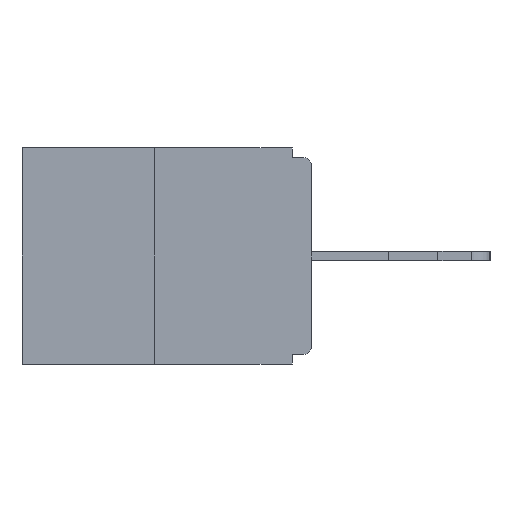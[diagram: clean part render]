
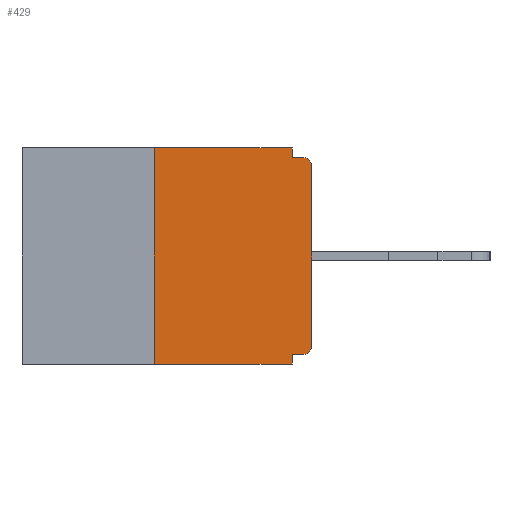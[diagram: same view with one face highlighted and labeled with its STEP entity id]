
A CAD part, left-side view. The second image highlights one B-rep face of the part: STEP entity #429.
In plain terms, the highlighted planar face has unit normal (-1, 0, 0).
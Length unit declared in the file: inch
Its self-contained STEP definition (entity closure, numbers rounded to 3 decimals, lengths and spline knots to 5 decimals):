
#134 = VERTEX_POINT ( 'NONE', #3484 ) ;
#415 = CARTESIAN_POINT ( 'NONE',  ( 0., 0.46, 0. ) ) ;
#429 = ADVANCED_FACE ( 'NONE', ( #4463 ), #9587, .F. ) ;
#510 = EDGE_CURVE ( 'NONE', #134, #20403, #24511, .T. ) ;
#675 = VECTOR ( 'NONE', #11992, 39.37008 ) ;
#1429 = DIRECTION ( 'NONE',  ( 1., 0., 0. ) ) ;
#1517 = DIRECTION ( 'NONE',  ( 0., 1., 0. ) ) ;
#1575 = EDGE_CURVE ( 'NONE', #20032, #6018, #9536, .T. ) ;
#1685 = CARTESIAN_POINT ( 'NONE',  ( 0., 0.46, -0.343 ) ) ;
#1712 = CARTESIAN_POINT ( 'NONE',  ( 0., 0.015, -0.313 ) ) ;
#1956 = CARTESIAN_POINT ( 'NONE',  ( 0., 0., -0.015 ) ) ;
#2131 = LINE ( 'NONE', #18532, #675 ) ;
#2180 = CARTESIAN_POINT ( 'NONE',  ( 0., 0., -0.313 ) ) ;
#2469 = EDGE_CURVE ( 'NONE', #26115, #7521, #4935, .T. ) ;
#3102 = DIRECTION ( 'NONE',  ( 0., -1., 0. ) ) ;
#3484 = CARTESIAN_POINT ( 'NONE',  ( 0., 0., -0.03 ) ) ;
#3559 = VECTOR ( 'NONE', #7073, 39.37008 ) ;
#4042 = DIRECTION ( 'NONE',  ( 0., 0., -1. ) ) ;
#4463 = FACE_OUTER_BOUND ( 'NONE', #23758, .T. ) ;
#4718 = LINE ( 'NONE', #1956, #21515 ) ;
#4935 = LINE ( 'NONE', #19039, #9870 ) ;
#4983 = ORIENTED_EDGE ( 'NONE', *, *, #21768, .T. ) ;
#4991 = VERTEX_POINT ( 'NONE', #2180 ) ;
#5872 = CARTESIAN_POINT ( 'NONE',  ( 0., 0.031, 0. ) ) ;
#6018 = VERTEX_POINT ( 'NONE', #18554 ) ;
#6286 = ORIENTED_EDGE ( 'NONE', *, *, #24197, .T. ) ;
#6769 = EDGE_CURVE ( 'NONE', #26792, #20403, #4718, .T. ) ;
#6835 = ORIENTED_EDGE ( 'NONE', *, *, #510, .T. ) ;
#6921 = EDGE_CURVE ( 'NONE', #4991, #134, #27020, .T. ) ;
#7037 = ORIENTED_EDGE ( 'NONE', *, *, #6769, .F. ) ;
#7073 = DIRECTION ( 'NONE',  ( 0., 0., -1. ) ) ;
#7521 = VERTEX_POINT ( 'NONE', #11473 ) ;
#8380 = CARTESIAN_POINT ( 'NONE',  ( 0., 0., -0.328 ) ) ;
#9536 = LINE ( 'NONE', #11171, #3559 ) ;
#9587 = PLANE ( 'NONE',  #10452 ) ;
#9870 = VECTOR ( 'NONE', #21928, 39.37008 ) ;
#10041 = ORIENTED_EDGE ( 'NONE', *, *, #2469, .F. ) ;
#10452 = AXIS2_PLACEMENT_3D ( 'NONE', #415, #1429, #25728 ) ;
#10807 = ORIENTED_EDGE ( 'NONE', *, *, #24813, .F. ) ;
#11171 = CARTESIAN_POINT ( 'NONE',  ( 0., 0.031, -0.343 ) ) ;
#11473 = CARTESIAN_POINT ( 'NONE',  ( 0., 0.25, 0. ) ) ;
#11699 = CARTESIAN_POINT ( 'NONE',  ( 0., 0.031, -0.328 ) ) ;
#11858 = ORIENTED_EDGE ( 'NONE', *, *, #15139, .F. ) ;
#11992 = DIRECTION ( 'NONE',  ( 0., -1., 0. ) ) ;
#13559 = ORIENTED_EDGE ( 'NONE', *, *, #6921, .T. ) ;
#13993 = VERTEX_POINT ( 'NONE', #5872 ) ;
#14377 = AXIS2_PLACEMENT_3D ( 'NONE', #1712, #17237, #4042 ) ;
#14824 = AXIS2_PLACEMENT_3D ( 'NONE', #27119, #28222, #25257 ) ;
#15139 = EDGE_CURVE ( 'NONE', #7521, #13993, #2131, .T. ) ;
#15173 = CARTESIAN_POINT ( 'NONE',  ( 0., 0.25, -0.343 ) ) ;
#15733 = VECTOR ( 'NONE', #1517, 39.37008 ) ;
#16503 = LINE ( 'NONE', #23653, #27327 ) ;
#17237 = DIRECTION ( 'NONE',  ( -1., 0., 0. ) ) ;
#18532 = CARTESIAN_POINT ( 'NONE',  ( 0., 0.46, 0. ) ) ;
#18554 = CARTESIAN_POINT ( 'NONE',  ( 0., 0.031, -0.343 ) ) ;
#19039 = CARTESIAN_POINT ( 'NONE',  ( 0., 0.25, 0. ) ) ;
#19692 = CARTESIAN_POINT ( 'NONE',  ( 0., 0.031, -0.015 ) ) ;
#20016 = ORIENTED_EDGE ( 'NONE', *, *, #20927, .F. ) ;
#20032 = VERTEX_POINT ( 'NONE', #11699 ) ;
#20403 = VERTEX_POINT ( 'NONE', #21704 ) ;
#20927 = EDGE_CURVE ( 'NONE', #26843, #20032, #27241, .T. ) ;
#21291 = VECTOR ( 'NONE', #22231, 39.37008 ) ;
#21306 = VECTOR ( 'NONE', #23831, 39.37008 ) ;
#21515 = VECTOR ( 'NONE', #3102, 39.37008 ) ;
#21704 = CARTESIAN_POINT ( 'NONE',  ( 0., 0.015, -0.015 ) ) ;
#21768 = EDGE_CURVE ( 'NONE', #26843, #4991, #25808, .T. ) ;
#21928 = DIRECTION ( 'NONE',  ( 0., 0., 1. ) ) ;
#22231 = DIRECTION ( 'NONE',  ( 0., 0., 1. ) ) ;
#22406 = CARTESIAN_POINT ( 'NONE',  ( 0., 0., 0. ) ) ;
#23653 = CARTESIAN_POINT ( 'NONE',  ( 0., 0.031, 0. ) ) ;
#23758 = EDGE_LOOP ( 'NONE', ( #11858, #10041, #6286, #27606, #20016, #4983, #13559, #6835, #7037, #10807 ) ) ;
#23831 = DIRECTION ( 'NONE',  ( 0., -1., 0. ) ) ;
#24197 = EDGE_CURVE ( 'NONE', #26115, #6018, #27695, .T. ) ;
#24511 = CIRCLE ( 'NONE', #14824, 0.015 ) ;
#24813 = EDGE_CURVE ( 'NONE', #13993, #26792, #16503, .T. ) ;
#25257 = DIRECTION ( 'NONE',  ( 0., 0., -1. ) ) ;
#25728 = DIRECTION ( 'NONE',  ( 0., 0., -1. ) ) ;
#25808 = CIRCLE ( 'NONE', #14377, 0.015 ) ;
#26115 = VERTEX_POINT ( 'NONE', #15173 ) ;
#26352 = CARTESIAN_POINT ( 'NONE',  ( 0., 0.015, -0.328 ) ) ;
#26792 = VERTEX_POINT ( 'NONE', #19692 ) ;
#26843 = VERTEX_POINT ( 'NONE', #26352 ) ;
#27020 = LINE ( 'NONE', #22406, #21291 ) ;
#27119 = CARTESIAN_POINT ( 'NONE',  ( 0., 0.015, -0.03 ) ) ;
#27241 = LINE ( 'NONE', #8380, #15733 ) ;
#27327 = VECTOR ( 'NONE', #27872, 39.37008 ) ;
#27606 = ORIENTED_EDGE ( 'NONE', *, *, #1575, .F. ) ;
#27695 = LINE ( 'NONE', #1685, #21306 ) ;
#27872 = DIRECTION ( 'NONE',  ( 0., 0., -1. ) ) ;
#28222 = DIRECTION ( 'NONE',  ( -1., 0., 0. ) ) ;
